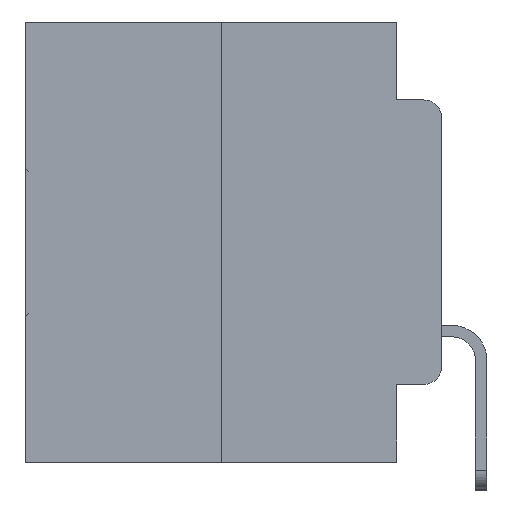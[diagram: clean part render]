
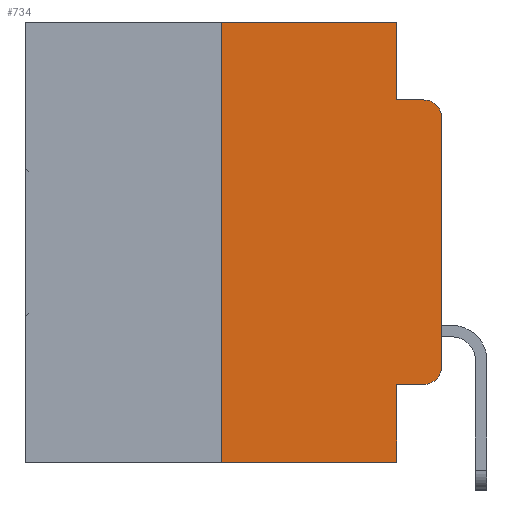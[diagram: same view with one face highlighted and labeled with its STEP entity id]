
A CAD part, left-side view. The second image highlights one B-rep face of the part: STEP entity #734.
In plain terms, the highlighted planar face has unit normal (-1, 0, 0).
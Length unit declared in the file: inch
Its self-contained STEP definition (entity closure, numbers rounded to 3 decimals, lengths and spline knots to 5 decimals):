
#242 = AXIS2_PLACEMENT_3D ( 'NONE', #8909, #11502, #27979 ) ;
#734 = ADVANCED_FACE ( 'NONE', ( #12442 ), #9034, .F. ) ;
#1012 = LINE ( 'NONE', #7149, #21603 ) ;
#1038 = CARTESIAN_POINT ( 'NONE',  ( 0., 0.02, -0.1085 ) ) ;
#1124 = DIRECTION ( 'NONE',  ( -1., 0., 0. ) ) ;
#1207 = CARTESIAN_POINT ( 'NONE',  ( 0., 0.25, 0. ) ) ;
#1537 = AXIS2_PLACEMENT_3D ( 'NONE', #1038, #18528, #3865 ) ;
#2202 = CIRCLE ( 'NONE', #1537, 0.02 ) ;
#2274 = VERTEX_POINT ( 'NONE', #20467 ) ;
#2287 = EDGE_CURVE ( 'NONE', #20734, #19579, #11482, .T. ) ;
#3238 = DIRECTION ( 'NONE',  ( 0., 0., 1. ) ) ;
#3865 = DIRECTION ( 'NONE',  ( 0., 0., -1. ) ) ;
#4069 = CARTESIAN_POINT ( 'NONE',  ( 0., 0.25, 0. ) ) ;
#4130 = EDGE_CURVE ( 'NONE', #2274, #20734, #17021, .T. ) ;
#4179 = CARTESIAN_POINT ( 'NONE',  ( 0., 0.051, -0.5 ) ) ;
#4541 = VERTEX_POINT ( 'NONE', #15930 ) ;
#4887 = VECTOR ( 'NONE', #16249, 39.37008 ) ;
#4987 = VERTEX_POINT ( 'NONE', #12557 ) ;
#5648 = VECTOR ( 'NONE', #8982, 39.37008 ) ;
#5891 = EDGE_CURVE ( 'NONE', #2274, #30022, #24753, .T. ) ;
#6352 = VECTOR ( 'NONE', #27854, 39.37008 ) ;
#6395 = CARTESIAN_POINT ( 'NONE',  ( 0., 0.051, 0. ) ) ;
#7148 = VERTEX_POINT ( 'NONE', #30703 ) ;
#7149 = CARTESIAN_POINT ( 'NONE',  ( 0., 0.473, 0. ) ) ;
#7282 = EDGE_LOOP ( 'NONE', ( #10987, #13936, #21825, #16141, #8311, #9877, #19966, #22248, #30312, #29288 ) ) ;
#7379 = EDGE_CURVE ( 'NONE', #4541, #30022, #18175, .T. ) ;
#8222 = CARTESIAN_POINT ( 'NONE',  ( 0., 0.473, -0.5 ) ) ;
#8311 = ORIENTED_EDGE ( 'NONE', *, *, #23336, .F. ) ;
#8716 = VERTEX_POINT ( 'NONE', #8894 ) ;
#8894 = CARTESIAN_POINT ( 'NONE',  ( 0., 0.02, -0.0885 ) ) ;
#8909 = CARTESIAN_POINT ( 'NONE',  ( 0., 0.473, 0. ) ) ;
#8982 = DIRECTION ( 'NONE',  ( 0., -1., 0. ) ) ;
#9034 = PLANE ( 'NONE',  #242 ) ;
#9257 = EDGE_CURVE ( 'NONE', #4541, #29963, #16942, .T. ) ;
#9877 = ORIENTED_EDGE ( 'NONE', *, *, #9257, .F. ) ;
#10671 = VECTOR ( 'NONE', #13953, 39.37008 ) ;
#10893 = EDGE_CURVE ( 'NONE', #4987, #7148, #29974, .T. ) ;
#10987 = ORIENTED_EDGE ( 'NONE', *, *, #15616, .T. ) ;
#11268 = VECTOR ( 'NONE', #16135, 39.37008 ) ;
#11482 = CIRCLE ( 'NONE', #23419, 0.02 ) ;
#11502 = DIRECTION ( 'NONE',  ( 1., 0., 0. ) ) ;
#11876 = VECTOR ( 'NONE', #24931, 39.37008 ) ;
#12123 = LINE ( 'NONE', #15442, #25473 ) ;
#12292 = LINE ( 'NONE', #28026, #4887 ) ;
#12442 = FACE_OUTER_BOUND ( 'NONE', #7282, .T. ) ;
#12502 = EDGE_CURVE ( 'NONE', #7148, #8716, #12292, .T. ) ;
#12557 = CARTESIAN_POINT ( 'NONE',  ( 0., 0.051, 0. ) ) ;
#13936 = ORIENTED_EDGE ( 'NONE', *, *, #14061, .T. ) ;
#13953 = DIRECTION ( 'NONE',  ( 0., 0., 1. ) ) ;
#14061 = EDGE_CURVE ( 'NONE', #30942, #8716, #2202, .T. ) ;
#15442 = CARTESIAN_POINT ( 'NONE',  ( 0., 0., 0. ) ) ;
#15616 = EDGE_CURVE ( 'NONE', #19579, #30942, #12123, .T. ) ;
#15930 = CARTESIAN_POINT ( 'NONE',  ( 0., 0.25, -0.5 ) ) ;
#16135 = DIRECTION ( 'NONE',  ( 0., 0., -1. ) ) ;
#16141 = ORIENTED_EDGE ( 'NONE', *, *, #10893, .F. ) ;
#16153 = CARTESIAN_POINT ( 'NONE',  ( 0., 0.02, -0.3915 ) ) ;
#16249 = DIRECTION ( 'NONE',  ( 0., -1., 0. ) ) ;
#16942 = LINE ( 'NONE', #1207, #10671 ) ;
#17021 = LINE ( 'NONE', #23341, #5648 ) ;
#18175 = LINE ( 'NONE', #8222, #11876 ) ;
#18528 = DIRECTION ( 'NONE',  ( -1., 0., 0. ) ) ;
#18591 = DIRECTION ( 'NONE',  ( 0., 0., -1. ) ) ;
#19579 = VERTEX_POINT ( 'NONE', #27374 ) ;
#19966 = ORIENTED_EDGE ( 'NONE', *, *, #7379, .T. ) ;
#20467 = CARTESIAN_POINT ( 'NONE',  ( 0., 0.051, -0.4115 ) ) ;
#20734 = VERTEX_POINT ( 'NONE', #24120 ) ;
#21581 = DIRECTION ( 'NONE',  ( 0., -1., 0. ) ) ;
#21603 = VECTOR ( 'NONE', #21581, 39.37008 ) ;
#21825 = ORIENTED_EDGE ( 'NONE', *, *, #12502, .F. ) ;
#22248 = ORIENTED_EDGE ( 'NONE', *, *, #5891, .F. ) ;
#23336 = EDGE_CURVE ( 'NONE', #29963, #4987, #1012, .T. ) ;
#23341 = CARTESIAN_POINT ( 'NONE',  ( 0., 0.051, -0.4115 ) ) ;
#23419 = AXIS2_PLACEMENT_3D ( 'NONE', #16153, #1124, #18591 ) ;
#24120 = CARTESIAN_POINT ( 'NONE',  ( 0., 0.02, -0.4115 ) ) ;
#24753 = LINE ( 'NONE', #6395, #6352 ) ;
#24931 = DIRECTION ( 'NONE',  ( 0., -1., 0. ) ) ;
#25473 = VECTOR ( 'NONE', #3238, 39.37008 ) ;
#27374 = CARTESIAN_POINT ( 'NONE',  ( 0., 0., -0.3915 ) ) ;
#27854 = DIRECTION ( 'NONE',  ( 0., 0., -1. ) ) ;
#27902 = CARTESIAN_POINT ( 'NONE',  ( 0., 0.051, 0. ) ) ;
#27979 = DIRECTION ( 'NONE',  ( 0., 0., -1. ) ) ;
#28026 = CARTESIAN_POINT ( 'NONE',  ( 0., 0.051, -0.0885 ) ) ;
#29288 = ORIENTED_EDGE ( 'NONE', *, *, #2287, .T. ) ;
#29380 = CARTESIAN_POINT ( 'NONE',  ( 0., 0., -0.1085 ) ) ;
#29963 = VERTEX_POINT ( 'NONE', #4069 ) ;
#29974 = LINE ( 'NONE', #27902, #11268 ) ;
#30022 = VERTEX_POINT ( 'NONE', #4179 ) ;
#30312 = ORIENTED_EDGE ( 'NONE', *, *, #4130, .T. ) ;
#30703 = CARTESIAN_POINT ( 'NONE',  ( 0., 0.051, -0.0885 ) ) ;
#30942 = VERTEX_POINT ( 'NONE', #29380 ) ;
